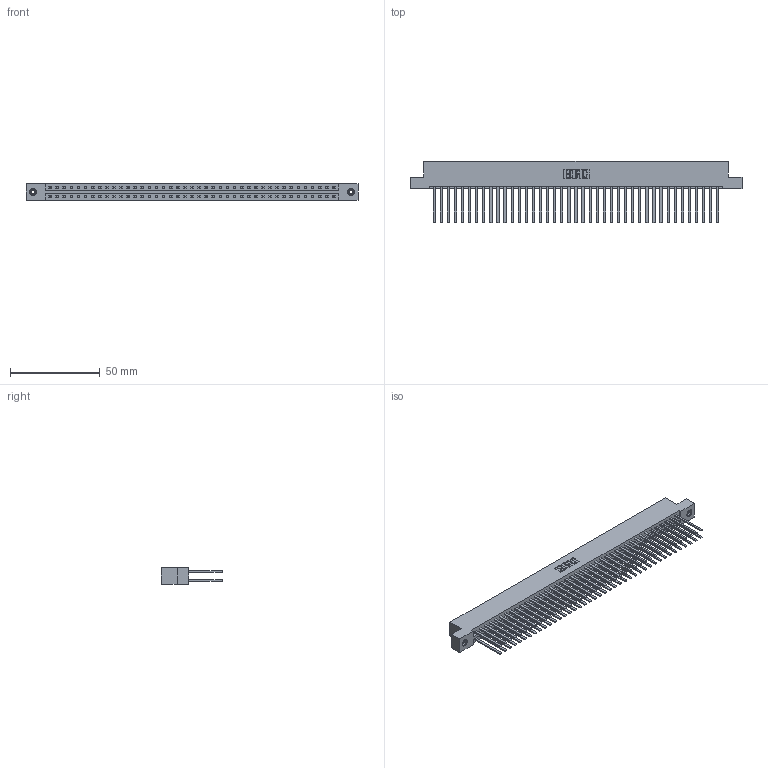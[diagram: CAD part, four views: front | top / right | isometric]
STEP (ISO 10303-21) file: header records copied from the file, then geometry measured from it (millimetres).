
FILE_DESCRIPTION (( 'STEP AP203' ), '1' );
FILE_NAME ('387-082-544-208.STEP', '2019-10-22T23:58:50', ( '' ), ( '' ), 'SwSTEP 2.0', 'SolidWorks 2016', '' );
FILE_SCHEMA (( 'CONFIG_CONTROL_DESIGN' ));
Length unit declared in the file: inch
Products named in the file (4): 345-250-001_345-250-003-102; 387-082-544-208; 337 Part_Flush Mounting Lugs - 0.156 Dia-TI; 345-292-001_345-293-144
Assembly tree (85 placements, depth 2):
  387-082-544-208
    337 Part_Flush Mounting Lugs - 0.156 Dia-TI
    345-292-001_345-293-144  x82
    345-250-001_345-250-003-102  x2
Bounding box: 185.47 x 34.3 x 9.4 mm (x, y, z)
Volume: 20676 mm3; surface area: 27143.6 mm2
Topology: 85 solids, 85 shells, 4110 faces, 12173 edges, 7998 vertices
Faces by surface type: plane 2890, cylinder 1204, cone 12, torus 4
Entity records: 32920 total; most frequent: CARTESIAN_POINT 5525, ORIENTED_EDGE 5454, DIRECTION 4729, EDGE_CURVE 2727, LINE 2583, VECTOR 2583, VERTEX_POINT 1812, AXIS2_PLACEMENT_3D 1073
